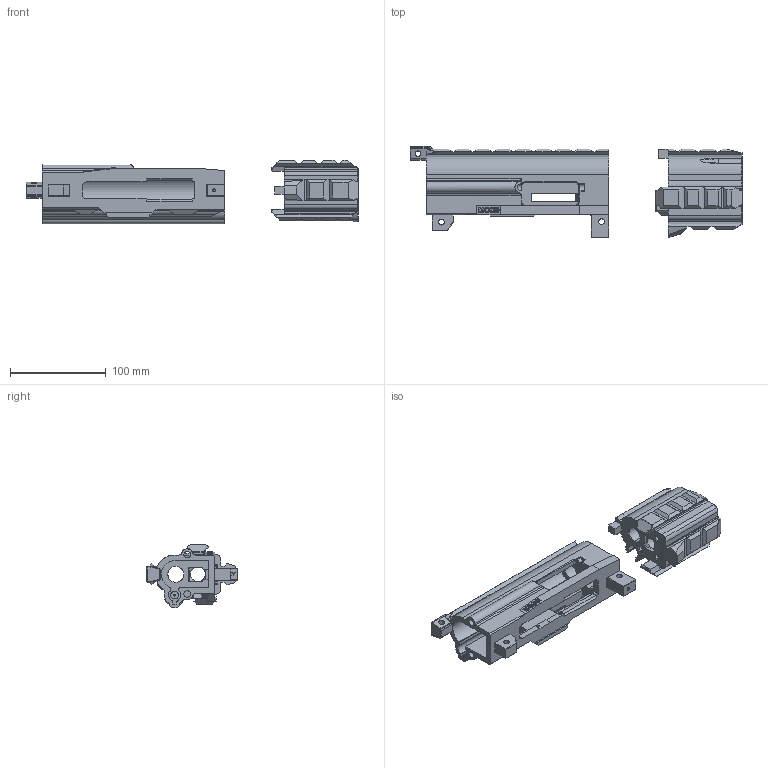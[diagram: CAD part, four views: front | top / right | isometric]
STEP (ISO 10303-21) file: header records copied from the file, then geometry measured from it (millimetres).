
FILE_DESCRIPTION(('STEP AP214'),'1');
FILE_NAME('MOD9 SW9VE Set v2.0.stp','2020-10-10T22:48:09',(' '),(' '),'Spatial InterOp 3D',' ',' ');
FILE_SCHEMA(('AUTOMOTIVE_DESIGN { 1 0 10303 214 1 1 1 1 }'));
Length unit declared in the file: metre
Products named in the file (3): MOD9 SW9VE Set v2.0; MOD9 SW9VE Upper Receiver Final; MOD9 SW9VE Barrel Retainer Final
Assembly tree (2 placements, depth 2):
  MOD9 SW9VE Set v2.0
    MOD9 SW9VE Upper Receiver Final
    MOD9 SW9VE Barrel Retainer Final
Bounding box: 346.21 x 94.9 x 65.85 mm (x, y, z)
Volume: 411199.2 mm3; surface area: 136754.2 mm2
Topology: 2 solids, 2 shells, 1344 faces, 3683 edges, 2371 vertices
Faces by surface type: plane 590, cylinder 369, bspline 220, cone 93, torus 34, extrusion 30, sphere 8
Entity records: 47177 total; most frequent: CARTESIAN_POINT 14347, ORIENTED_EDGE 7358, DIRECTION 6022, EDGE_CURVE 3679, VERTEX_POINT 2371, VECTOR 2186, LINE 2156, AXIS2_PLACEMENT_3D 1918
